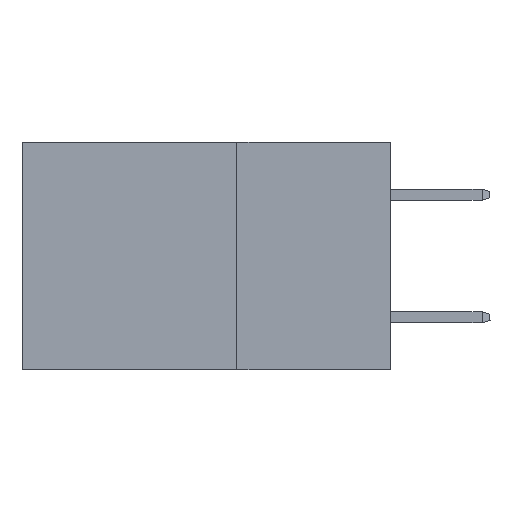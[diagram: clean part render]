
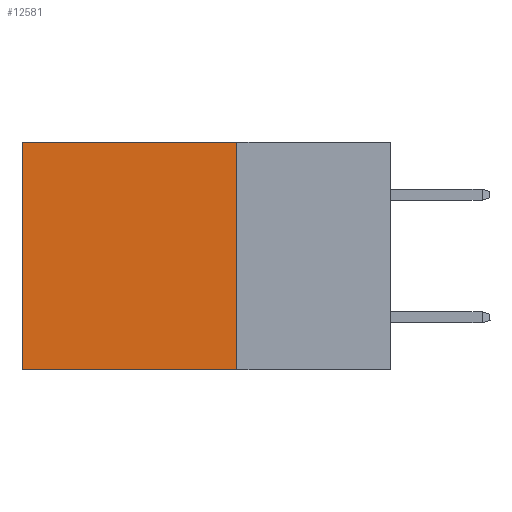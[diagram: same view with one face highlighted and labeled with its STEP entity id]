
A CAD part, left-side view. The second image highlights one B-rep face of the part: STEP entity #12581.
In plain terms, the highlighted planar face has unit normal (-1, 0, 0).
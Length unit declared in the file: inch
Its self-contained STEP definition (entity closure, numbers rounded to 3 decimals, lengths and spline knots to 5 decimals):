
#593 = EDGE_CURVE ( 'NONE', #23327, #30000, #12004, .T. ) ;
#976 = DIRECTION ( 'NONE',  ( 0., 0., -1. ) ) ;
#3299 = ORIENTED_EDGE ( 'NONE', *, *, #11306, .F. ) ;
#3357 = CARTESIAN_POINT ( 'NONE',  ( 0.2875, 0.25, 0. ) ) ;
#3424 = VECTOR ( 'NONE', #13701, 39.37008 ) ;
#3707 = CARTESIAN_POINT ( 'NONE',  ( 0.2875, 0.6, 0. ) ) ;
#4435 = LINE ( 'NONE', #3357, #24389 ) ;
#8449 = ORIENTED_EDGE ( 'NONE', *, *, #593, .F. ) ;
#8861 = CARTESIAN_POINT ( 'NONE',  ( 0.2875, 0.6, -0.37 ) ) ;
#10631 = DIRECTION ( 'NONE',  ( 0., 1., 0. ) ) ;
#10873 = CARTESIAN_POINT ( 'NONE',  ( 0.2875, 0.25, 0. ) ) ;
#11306 = EDGE_CURVE ( 'NONE', #30000, #29849, #13649, .T. ) ;
#12004 = LINE ( 'NONE', #20941, #23317 ) ;
#12581 = ADVANCED_FACE ( 'NONE', ( #25595 ), #25258, .F. ) ;
#13050 = DIRECTION ( 'NONE',  ( 1., 0., 0. ) ) ;
#13485 = EDGE_CURVE ( 'NONE', #23327, #23137, #4435, .T. ) ;
#13620 = CARTESIAN_POINT ( 'NONE',  ( 0.2875, 0.6, 0. ) ) ;
#13649 = LINE ( 'NONE', #19051, #14378 ) ;
#13701 = DIRECTION ( 'NONE',  ( 0., 0., -1. ) ) ;
#14378 = VECTOR ( 'NONE', #17090, 39.37008 ) ;
#16203 = ORIENTED_EDGE ( 'NONE', *, *, #13485, .T. ) ;
#16342 = EDGE_CURVE ( 'NONE', #23137, #29849, #20769, .T. ) ;
#16385 = DIRECTION ( 'NONE',  ( 0., 0., -1. ) ) ;
#17090 = DIRECTION ( 'NONE',  ( 0., 1., 0. ) ) ;
#19051 = CARTESIAN_POINT ( 'NONE',  ( 0.2875, 0.25, -0.37 ) ) ;
#20769 = LINE ( 'NONE', #3707, #3424 ) ;
#20941 = CARTESIAN_POINT ( 'NONE',  ( 0.2875, 0.25, 0. ) ) ;
#21666 = ORIENTED_EDGE ( 'NONE', *, *, #16342, .T. ) ;
#23137 = VERTEX_POINT ( 'NONE', #13620 ) ;
#23317 = VECTOR ( 'NONE', #16385, 39.37008 ) ;
#23327 = VERTEX_POINT ( 'NONE', #26143 ) ;
#24389 = VECTOR ( 'NONE', #10631, 39.37008 ) ;
#24753 = EDGE_LOOP ( 'NONE', ( #21666, #3299, #8449, #16203 ) ) ;
#24769 = AXIS2_PLACEMENT_3D ( 'NONE', #10873, #13050, #976 ) ;
#25258 = PLANE ( 'NONE',  #24769 ) ;
#25595 = FACE_OUTER_BOUND ( 'NONE', #24753, .T. ) ;
#26143 = CARTESIAN_POINT ( 'NONE',  ( 0.2875, 0.25, 0. ) ) ;
#29849 = VERTEX_POINT ( 'NONE', #8861 ) ;
#30000 = VERTEX_POINT ( 'NONE', #30901 ) ;
#30901 = CARTESIAN_POINT ( 'NONE',  ( 0.2875, 0.25, -0.37 ) ) ;
